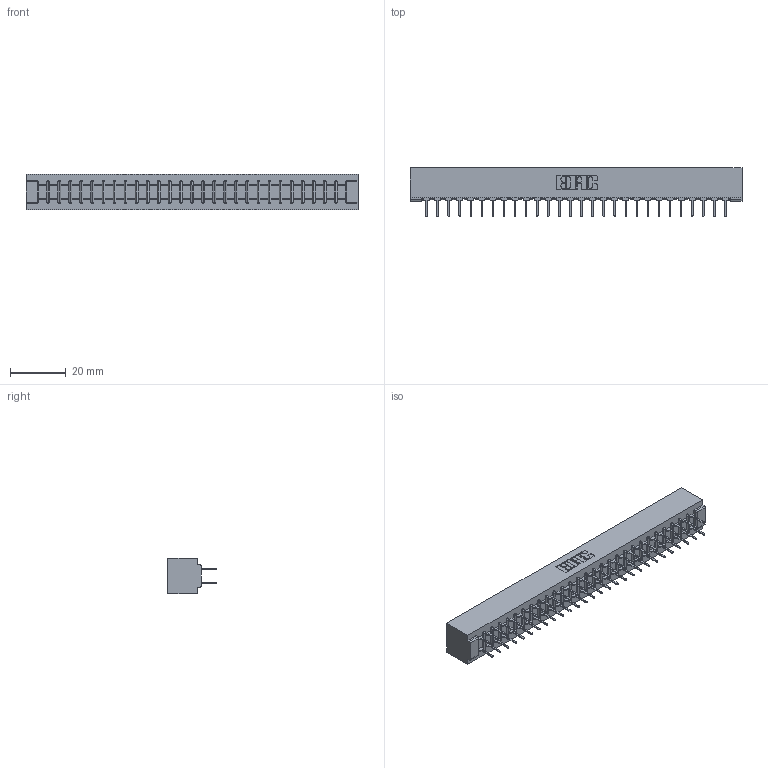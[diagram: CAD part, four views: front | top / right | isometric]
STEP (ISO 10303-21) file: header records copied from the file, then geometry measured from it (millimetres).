
FILE_DESCRIPTION (( 'STEP AP203' ), '1' );
FILE_NAME ('357-056-524-201.STEP', '2019-09-19T04:35:51', ( '' ), ( '' ), 'SwSTEP 2.0', 'SolidWorks 2016', '' );
FILE_SCHEMA (( 'CONFIG_CONTROL_DESIGN' ));
Length unit declared in the file: inch
Products named in the file (3): 307 Part_No Mounting Lugs; 357-056-524-201; 307-290-001_524
Assembly tree (57 placements, depth 2):
  357-056-524-201
    307 Part_No Mounting Lugs
    307-290-001_524  x56
Bounding box: 118.82 x 17.42 x 12.7 mm (x, y, z)
Volume: 13065.5 mm3; surface area: 15827.4 mm2
Topology: 57 solids, 57 shells, 2715 faces, 7579 edges, 4898 vertices
Faces by surface type: plane 1802, cylinder 855, sphere 58
Entity records: 26316 total; most frequent: CARTESIAN_POINT 4304, ORIENTED_EDGE 4262, DIRECTION 4221, EDGE_CURVE 2131, LINE 1631, VECTOR 1631, VERTEX_POINT 1378, AXIS2_PLACEMENT_3D 1295
